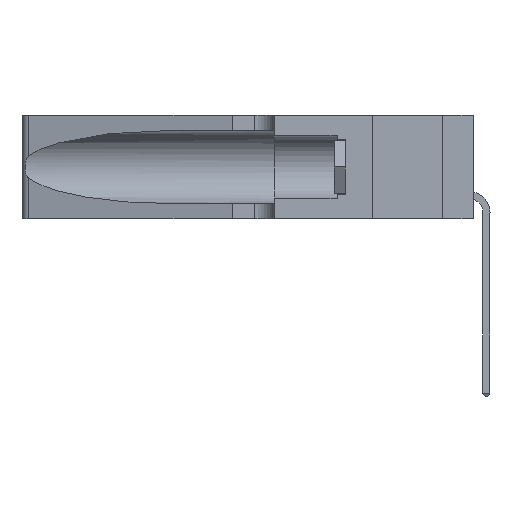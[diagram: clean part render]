
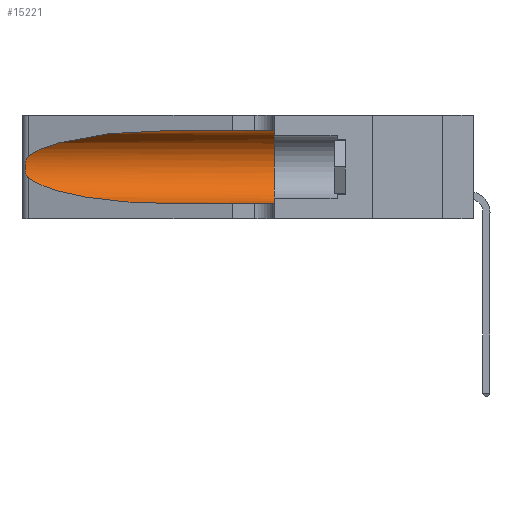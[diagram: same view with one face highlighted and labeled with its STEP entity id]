
A CAD part, left-side view. The second image highlights one B-rep face of the part: STEP entity #15221.
In plain terms, the highlighted cylindrical face has radius 3.308 mm (diameter 6.617 mm), a partial arc.
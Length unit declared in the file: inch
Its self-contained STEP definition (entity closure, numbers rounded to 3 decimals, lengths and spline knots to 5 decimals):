
#2355 = CARTESIAN_POINT ( 'NONE',  ( 0.25789, 1.23486, 0.15765 ) ) ;
#2433 = EDGE_CURVE ( 'NONE', #16645, #22509, #4045, .T. ) ;
#2497 = VERTEX_POINT ( 'NONE', #25598 ) ;
#2987 = CARTESIAN_POINT ( 'NONE',  ( 0.1305, 1.61858, 0.31525 ) ) ;
#3338 = CARTESIAN_POINT ( 'NONE',  ( 0.1305, 0.35, 0.05475 ) ) ;
#4045 = LINE ( 'NONE', #5193, #26432 ) ;
#5004 = CARTESIAN_POINT ( 'NONE',  ( 0.25487, 1.22718, 0.22369 ) ) ;
#5193 = CARTESIAN_POINT ( 'NONE',  ( 0.1305, 1.61858, 0.05475 ) ) ;
#5239 = CARTESIAN_POINT ( 'NONE',  ( 0.25639, 1.23184, 0.21858 ) ) ;
#5387 = CARTESIAN_POINT ( 'NONE',  ( 0.2373, 1.15595, 0.28018 ) ) ;
#7123 = CARTESIAN_POINT ( 'NONE',  ( 0.1305, 0.72297, 0.05475 ) ) ;
#7757 = EDGE_CURVE ( 'NONE', #28625, #20493, #21060, .T. ) ;
#7843 =( BOUNDED_CURVE ( )  B_SPLINE_CURVE ( 3, ( #27970, #25538, #5387, #5004 ),
 .UNSPECIFIED., .F., .T. ) 
 B_SPLINE_CURVE_WITH_KNOTS ( ( 4, 4 ),
 ( 1.5708, 2.84003 ),
 .UNSPECIFIED. ) 
 CURVE ( )  GEOMETRIC_REPRESENTATION_ITEM ( )  RATIONAL_B_SPLINE_CURVE ( ( 1., 0.87, 0.87, 1. ) ) 
 REPRESENTATION_ITEM ( '' )  );
#8215 = CARTESIAN_POINT ( 'NONE',  ( 0.26075, 1.23896, 0.19203 ) ) ;
#8343 = CARTESIAN_POINT ( 'NONE',  ( 0.1305, 0.72297, 0.31525 ) ) ;
#8693 = DIRECTION ( 'NONE',  ( 0., -1., 0. ) ) ;
#9160 = ORIENTED_EDGE ( 'NONE', *, *, #31691, .T. ) ;
#9552 = EDGE_CURVE ( 'NONE', #28625, #10280, #7843, .T. ) ;
#10280 = VERTEX_POINT ( 'NONE', #36723 ) ;
#10830 = CARTESIAN_POINT ( 'NONE',  ( 0.25856, 1.23593, 0.16098 ) ) ;
#11082 = CARTESIAN_POINT ( 'NONE',  ( 0.25555, 1.22993, 0.14849 ) ) ;
#11181 = EDGE_CURVE ( 'NONE', #20493, #22509, #23884, .T. ) ;
#11312 = AXIS2_PLACEMENT_3D ( 'NONE', #31279, #22798, #28798 ) ;
#11682 =( BOUNDED_CURVE ( )  B_SPLINE_CURVE ( 3, ( #23221, #14803, #34713, #23720 ),
 .UNSPECIFIED., .F., .F. ) 
 B_SPLINE_CURVE_WITH_KNOTS ( ( 4, 4 ),
 ( 3.44316, 4.71239 ),
 .UNSPECIFIED. ) 
 CURVE ( )  GEOMETRIC_REPRESENTATION_ITEM ( )  RATIONAL_B_SPLINE_CURVE ( ( 1., 0.87, 0.87, 1. ) ) 
 REPRESENTATION_ITEM ( '' )  );
#13966 = CARTESIAN_POINT ( 'NONE',  ( 0.25487, 1.22718, 0.14631 ) ) ;
#14731 = AXIS2_PLACEMENT_3D ( 'NONE', #15863, #33014, #33282 ) ;
#14803 = CARTESIAN_POINT ( 'NONE',  ( 0.2373, 1.15595, 0.08982 ) ) ;
#15221 = ADVANCED_FACE ( 'NONE', ( #21611 ), #21117, .F. ) ;
#15863 = CARTESIAN_POINT ( 'NONE',  ( 0.1305, 1.61858, 0.185 ) ) ;
#16085 = ORIENTED_EDGE ( 'NONE', *, *, #36983, .T. ) ;
#16390 = CARTESIAN_POINT ( 'NONE',  ( 0.25854, 1.2359, 0.20912 ) ) ;
#16513 = CARTESIAN_POINT ( 'NONE',  ( 0.25787, 1.23484, 0.2124 ) ) ;
#16641 = CARTESIAN_POINT ( 'NONE',  ( 0.25555, 1.22994, 0.2215 ) ) ;
#16645 = VERTEX_POINT ( 'NONE', #7123 ) ;
#16951 = EDGE_LOOP ( 'NONE', ( #26297, #9160, #16085, #18986, #18737, #29867 ) ) ;
#18737 = ORIENTED_EDGE ( 'NONE', *, *, #11181, .F. ) ;
#18986 = ORIENTED_EDGE ( 'NONE', *, *, #2433, .T. ) ;
#19690 = CARTESIAN_POINT ( 'NONE',  ( 0.26018, 1.23835, 0.19895 ) ) ;
#20493 = VERTEX_POINT ( 'NONE', #32479 ) ;
#21060 = LINE ( 'NONE', #2987, #30897 ) ;
#21117 = CYLINDRICAL_SURFACE ( 'NONE', #14731, 0.13025 ) ;
#21155 = B_SPLINE_CURVE_WITH_KNOTS ( 'NONE', 3,
 ( #34309, #16641, #5239, #16513, #16390, #19690, #8215, #36528, #28073, #10830, #2355, #28330, #11082, #13966 ),
 .UNSPECIFIED., .F., .F.,
 ( 4, 2, 2, 2, 2, 2, 4 ),
 ( 0., 0.00027, 0.00053, 0.00107, 0.0016, 0.00187, 0.00214 ),
 .UNSPECIFIED. ) ;
#21611 = FACE_OUTER_BOUND ( 'NONE', #16951, .T. ) ;
#22509 = VERTEX_POINT ( 'NONE', #3338 ) ;
#22798 = DIRECTION ( 'NONE',  ( 0., 1., 0. ) ) ;
#23221 = CARTESIAN_POINT ( 'NONE',  ( 0.25487, 1.22718, 0.14631 ) ) ;
#23720 = CARTESIAN_POINT ( 'NONE',  ( 0.1305, 0.72297, 0.05475 ) ) ;
#23884 = CIRCLE ( 'NONE', #11312, 0.13025 ) ;
#25119 = DIRECTION ( 'NONE',  ( 0., -1., 0. ) ) ;
#25538 = CARTESIAN_POINT ( 'NONE',  ( 0.18966, 0.96281, 0.31525 ) ) ;
#25598 = CARTESIAN_POINT ( 'NONE',  ( 0.25487, 1.22718, 0.14631 ) ) ;
#26297 = ORIENTED_EDGE ( 'NONE', *, *, #9552, .T. ) ;
#26432 = VECTOR ( 'NONE', #25119, 39.37008 ) ;
#27970 = CARTESIAN_POINT ( 'NONE',  ( 0.1305, 0.72297, 0.31525 ) ) ;
#28073 = CARTESIAN_POINT ( 'NONE',  ( 0.26017, 1.23833, 0.17102 ) ) ;
#28330 = CARTESIAN_POINT ( 'NONE',  ( 0.25639, 1.23186, 0.15144 ) ) ;
#28625 = VERTEX_POINT ( 'NONE', #8343 ) ;
#28798 = DIRECTION ( 'NONE',  ( 0., 0., 1. ) ) ;
#29867 = ORIENTED_EDGE ( 'NONE', *, *, #7757, .F. ) ;
#30897 = VECTOR ( 'NONE', #8693, 39.37008 ) ;
#31279 = CARTESIAN_POINT ( 'NONE',  ( 0.1305, 0.35, 0.185 ) ) ;
#31691 = EDGE_CURVE ( 'NONE', #10280, #2497, #21155, .T. ) ;
#32479 = CARTESIAN_POINT ( 'NONE',  ( 0.1305, 0.35, 0.31525 ) ) ;
#33014 = DIRECTION ( 'NONE',  ( 0., -1., 0. ) ) ;
#33282 = DIRECTION ( 'NONE',  ( 0., 0., -1. ) ) ;
#34309 = CARTESIAN_POINT ( 'NONE',  ( 0.25487, 1.22718, 0.22369 ) ) ;
#34713 = CARTESIAN_POINT ( 'NONE',  ( 0.18966, 0.96281, 0.05475 ) ) ;
#36528 = CARTESIAN_POINT ( 'NONE',  ( 0.26075, 1.23896, 0.178 ) ) ;
#36723 = CARTESIAN_POINT ( 'NONE',  ( 0.25487, 1.22718, 0.22369 ) ) ;
#36983 = EDGE_CURVE ( 'NONE', #2497, #16645, #11682, .T. ) ;
